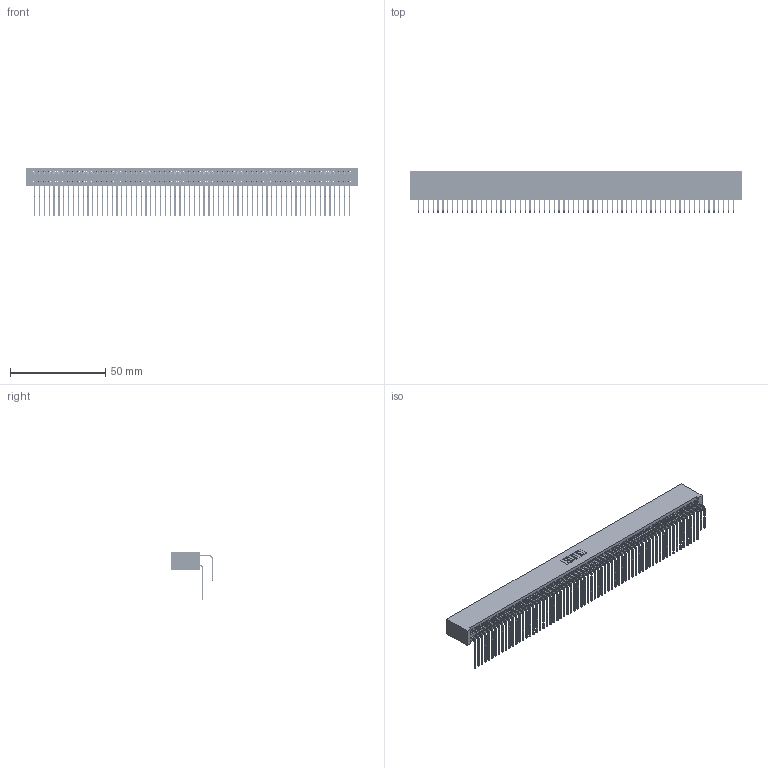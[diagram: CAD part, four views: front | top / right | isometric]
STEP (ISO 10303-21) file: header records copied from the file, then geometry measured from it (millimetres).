
FILE_DESCRIPTION (( 'STEP AP203' ), '1' );
FILE_NAME ('345-132-558-201.STEP', '2019-11-07T22:46:14', ( '' ), ( '' ), 'SwSTEP 2.0', 'SolidWorks 2016', '' );
FILE_SCHEMA (( 'CONFIG_CONTROL_DESIGN' ));
Length unit declared in the file: inch
Products named in the file (4): 345-132-558-201; 345-292-001_558 559 Tail - 1; 345-292-001_558 Tail - 2; 345 Part_No Mounting Lugs
Assembly tree (133 placements, depth 2):
  345-132-558-201
    345 Part_No Mounting Lugs
    345-292-001_558 559 Tail - 1  x66
    345-292-001_558 Tail - 2  x66
Bounding box: 174.24 x 21.83 x 25.53 mm (x, y, z)
Volume: 18526.4 mm3; surface area: 31733.9 mm2
Topology: 133 solids, 133 shells, 6982 faces, 20777 edges, 13674 vertices
Faces by surface type: plane 4696, cylinder 2286
Entity records: 49929 total; most frequent: CARTESIAN_POINT 8391, ORIENTED_EDGE 8274, DIRECTION 7337, EDGE_CURVE 4137, VECTOR 3709, LINE 3709, VERTEX_POINT 2754, AXIS2_PLACEMENT_3D 1814
